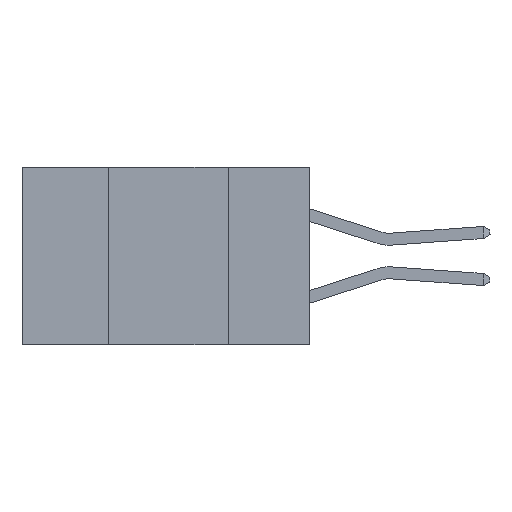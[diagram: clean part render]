
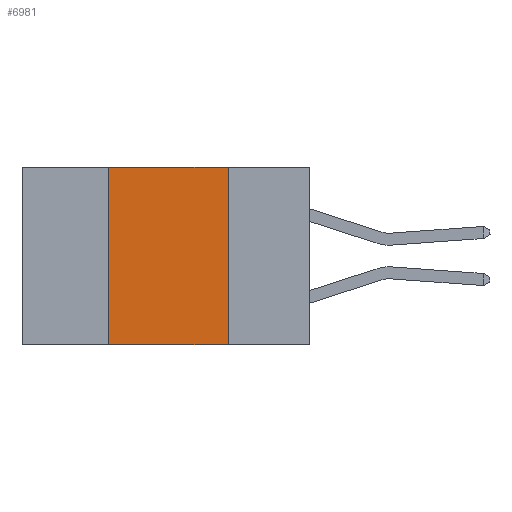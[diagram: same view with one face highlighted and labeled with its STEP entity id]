
A CAD part, left-side view. The second image highlights one B-rep face of the part: STEP entity #6981.
In plain terms, the highlighted planar face has unit normal (-1, 0, 0).
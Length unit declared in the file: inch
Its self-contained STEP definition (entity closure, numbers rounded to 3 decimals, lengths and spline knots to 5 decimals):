
#298 = LINE ( 'NONE', #4464, #9768 ) ;
#638 = CARTESIAN_POINT ( 'NONE',  ( 0., 0.42, 0. ) ) ;
#1037 = ORIENTED_EDGE ( 'NONE', *, *, #9099, .F. ) ;
#1246 = VECTOR ( 'NONE', #1714, 39.37008 ) ;
#1413 = EDGE_LOOP ( 'NONE', ( #11279, #10716, #1037, #10165 ) ) ;
#1714 = DIRECTION ( 'NONE',  ( 0., -1., 0. ) ) ;
#2254 = VERTEX_POINT ( 'NONE', #7374 ) ;
#2416 = CARTESIAN_POINT ( 'NONE',  ( 0., 0.17, -0.37 ) ) ;
#2928 = CARTESIAN_POINT ( 'NONE',  ( 0., 0.6, 0. ) ) ;
#3608 = EDGE_CURVE ( 'NONE', #9514, #2254, #10903, .T. ) ;
#4376 = DIRECTION ( 'NONE',  ( 0., 0., 1. ) ) ;
#4464 = CARTESIAN_POINT ( 'NONE',  ( 0., 0.42, -0.37 ) ) ;
#4734 = DIRECTION ( 'NONE',  ( 0., 0., -1. ) ) ;
#5026 = DIRECTION ( 'NONE',  ( 1., 0., 0. ) ) ;
#5264 = VERTEX_POINT ( 'NONE', #2416 ) ;
#5478 = PLANE ( 'NONE',  #5867 ) ;
#5504 = CARTESIAN_POINT ( 'NONE',  ( 0., 0.6, 0. ) ) ;
#5713 = CARTESIAN_POINT ( 'NONE',  ( 0., 0.6, -0.37 ) ) ;
#5867 = AXIS2_PLACEMENT_3D ( 'NONE', #5504, #5026, #4734 ) ;
#5998 = DIRECTION ( 'NONE',  ( 0., -1., 0. ) ) ;
#6395 = LINE ( 'NONE', #5713, #10888 ) ;
#6981 = ADVANCED_FACE ( 'NONE', ( #7042 ), #5478, .F. ) ;
#7042 = FACE_OUTER_BOUND ( 'NONE', #1413, .T. ) ;
#7374 = CARTESIAN_POINT ( 'NONE',  ( 0., 0.17, 0. ) ) ;
#8511 = VERTEX_POINT ( 'NONE', #10181 ) ;
#8923 = DIRECTION ( 'NONE',  ( 0., 0., -1. ) ) ;
#8958 = EDGE_CURVE ( 'NONE', #8511, #5264, #6395, .T. ) ;
#9099 = EDGE_CURVE ( 'NONE', #8511, #9514, #298, .T. ) ;
#9187 = CARTESIAN_POINT ( 'NONE',  ( 0., 0.17, -0.37 ) ) ;
#9201 = VECTOR ( 'NONE', #8923, 39.37008 ) ;
#9483 = LINE ( 'NONE', #9187, #9201 ) ;
#9514 = VERTEX_POINT ( 'NONE', #638 ) ;
#9631 = EDGE_CURVE ( 'NONE', #2254, #5264, #9483, .T. ) ;
#9768 = VECTOR ( 'NONE', #4376, 39.37008 ) ;
#10165 = ORIENTED_EDGE ( 'NONE', *, *, #8958, .T. ) ;
#10181 = CARTESIAN_POINT ( 'NONE',  ( 0., 0.42, -0.37 ) ) ;
#10716 = ORIENTED_EDGE ( 'NONE', *, *, #3608, .F. ) ;
#10888 = VECTOR ( 'NONE', #5998, 39.37008 ) ;
#10903 = LINE ( 'NONE', #2928, #1246 ) ;
#11279 = ORIENTED_EDGE ( 'NONE', *, *, #9631, .F. ) ;
